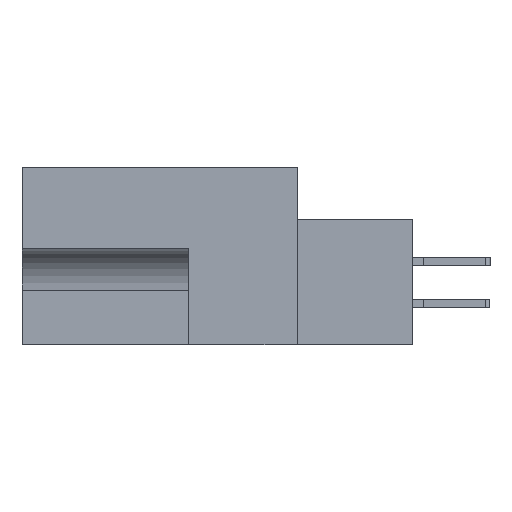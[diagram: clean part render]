
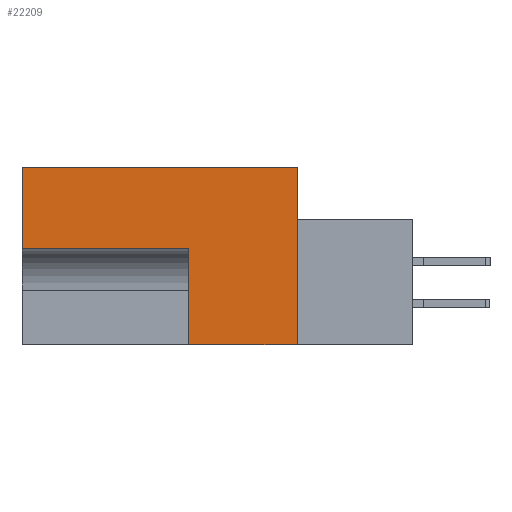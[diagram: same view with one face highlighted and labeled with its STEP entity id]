
A CAD part, left-side view. The second image highlights one B-rep face of the part: STEP entity #22209.
In plain terms, the highlighted planar face has unit normal (-1, 0, 0).
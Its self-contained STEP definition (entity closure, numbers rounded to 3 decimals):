
#591 = VERTEX_POINT ( 'NONE', #23223 ) ;
#1932 = DIRECTION ( 'NONE',  ( 0., 0., -1. ) ) ;
#3516 = VECTOR ( 'NONE', #17692, 1000. ) ;
#3875 = CARTESIAN_POINT ( 'NONE',  ( 0., 0., 0. ) ) ;
#4477 = CARTESIAN_POINT ( 'NONE',  ( 0., 11.506, 0. ) ) ;
#4665 = LINE ( 'NONE', #22205, #5241 ) ;
#5241 = VECTOR ( 'NONE', #18579, 1000. ) ;
#5518 = ORIENTED_EDGE ( 'NONE', *, *, #6550, .F. ) ;
#5524 = PLANE ( 'NONE',  #6151 ) ;
#5834 = VERTEX_POINT ( 'NONE', #19029 ) ;
#6072 = CARTESIAN_POINT ( 'NONE',  ( 0., 8.255, -13.487 ) ) ;
#6090 = CARTESIAN_POINT ( 'NONE',  ( 0., 0., -13.487 ) ) ;
#6151 = AXIS2_PLACEMENT_3D ( 'NONE', #3875, #12956, #1932 ) ;
#6157 = EDGE_CURVE ( 'NONE', #18762, #23318, #14992, .T. ) ;
#6228 = DIRECTION ( 'NONE',  ( 0., 0., 1. ) ) ;
#6233 = VECTOR ( 'NONE', #6228, 1000. ) ;
#6317 = CARTESIAN_POINT ( 'NONE',  ( 0., 0., 0. ) ) ;
#6439 = LINE ( 'NONE', #14982, #6714 ) ;
#6550 = EDGE_CURVE ( 'NONE', #11849, #591, #6439, .T. ) ;
#6560 = EDGE_LOOP ( 'NONE', ( #10897, #15942, #7531, #5518, #6825, #10643 ) ) ;
#6714 = VECTOR ( 'NONE', #22241, 1000. ) ;
#6825 = ORIENTED_EDGE ( 'NONE', *, *, #19081, .F. ) ;
#7285 = CARTESIAN_POINT ( 'NONE',  ( 0., 0., 0. ) ) ;
#7531 = ORIENTED_EDGE ( 'NONE', *, *, #11948, .F. ) ;
#10089 = DIRECTION ( 'NONE',  ( 0., -1., 0. ) ) ;
#10643 = ORIENTED_EDGE ( 'NONE', *, *, #14342, .F. ) ;
#10825 = LINE ( 'NONE', #15802, #3516 ) ;
#10897 = ORIENTED_EDGE ( 'NONE', *, *, #17336, .F. ) ;
#11471 = VERTEX_POINT ( 'NONE', #18380 ) ;
#11849 = VERTEX_POINT ( 'NONE', #23238 ) ;
#11948 = EDGE_CURVE ( 'NONE', #591, #18762, #15476, .T. ) ;
#12956 = DIRECTION ( 'NONE',  ( 1., 0., 0. ) ) ;
#14342 = EDGE_CURVE ( 'NONE', #5834, #11471, #16833, .T. ) ;
#14982 = CARTESIAN_POINT ( 'NONE',  ( 0., 20.955, -13.487 ) ) ;
#14992 = LINE ( 'NONE', #7285, #17645 ) ;
#15476 = LINE ( 'NONE', #4477, #17531 ) ;
#15802 = CARTESIAN_POINT ( 'NONE',  ( 0., -8.814, -13.487 ) ) ;
#15942 = ORIENTED_EDGE ( 'NONE', *, *, #6157, .F. ) ;
#16833 = LINE ( 'NONE', #6072, #6233 ) ;
#17336 = EDGE_CURVE ( 'NONE', #23318, #5834, #10825, .T. ) ;
#17531 = VECTOR ( 'NONE', #10089, 1000. ) ;
#17645 = VECTOR ( 'NONE', #24283, 1000. ) ;
#17692 = DIRECTION ( 'NONE',  ( 0., 1., 0. ) ) ;
#18380 = CARTESIAN_POINT ( 'NONE',  ( 0., 8.255, -6.172 ) ) ;
#18579 = DIRECTION ( 'NONE',  ( 0., 1., 0. ) ) ;
#18620 = FACE_OUTER_BOUND ( 'NONE', #6560, .T. ) ;
#18762 = VERTEX_POINT ( 'NONE', #6317 ) ;
#19029 = CARTESIAN_POINT ( 'NONE',  ( 0., 8.255, -13.487 ) ) ;
#19081 = EDGE_CURVE ( 'NONE', #11471, #11849, #4665, .T. ) ;
#22205 = CARTESIAN_POINT ( 'NONE',  ( 0., 8.255, -6.172 ) ) ;
#22209 = ADVANCED_FACE ( 'NONE', ( #18620 ), #5524, .F. ) ;
#22241 = DIRECTION ( 'NONE',  ( 0., 0., 1. ) ) ;
#23223 = CARTESIAN_POINT ( 'NONE',  ( 0., 20.955, 0. ) ) ;
#23238 = CARTESIAN_POINT ( 'NONE',  ( 0., 20.955, -6.172 ) ) ;
#23318 = VERTEX_POINT ( 'NONE', #6090 ) ;
#24283 = DIRECTION ( 'NONE',  ( 0., 0., -1. ) ) ;
